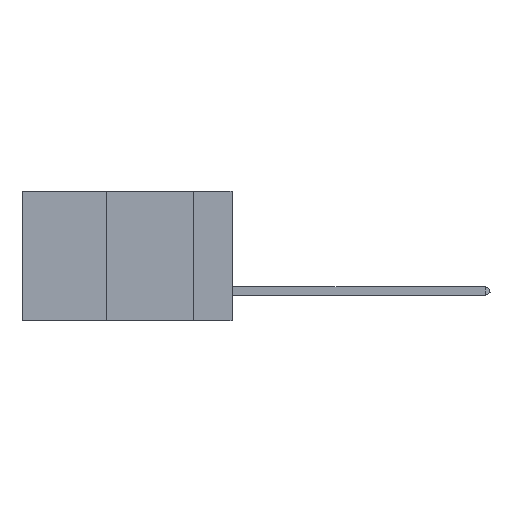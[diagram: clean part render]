
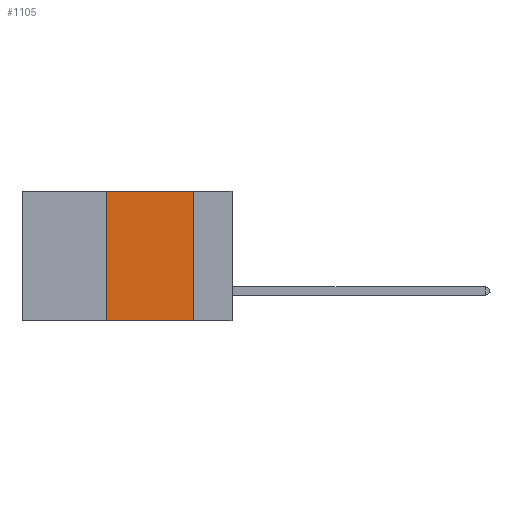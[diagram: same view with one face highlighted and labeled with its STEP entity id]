
A CAD part, left-side view. The second image highlights one B-rep face of the part: STEP entity #1105.
In plain terms, the highlighted planar face has unit normal (-1, 0, 0).
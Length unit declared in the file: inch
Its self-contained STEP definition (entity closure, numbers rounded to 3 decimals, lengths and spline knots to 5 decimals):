
#771 = CARTESIAN_POINT ( 'NONE',  ( 0., 0.6, -0.37 ) ) ;
#1045 = DIRECTION ( 'NONE',  ( 0., -1., 0. ) ) ;
#1105 = ADVANCED_FACE ( 'NONE', ( #7462 ), #9928, .F. ) ;
#1287 = CARTESIAN_POINT ( 'NONE',  ( 0., 0.36, 0. ) ) ;
#2020 = VERTEX_POINT ( 'NONE', #13612 ) ;
#2032 = CARTESIAN_POINT ( 'NONE',  ( 0., 0.11, -0.37 ) ) ;
#2173 = CARTESIAN_POINT ( 'NONE',  ( 0., 0.6, 0. ) ) ;
#2353 = LINE ( 'NONE', #771, #10437 ) ;
#2858 = DIRECTION ( 'NONE',  ( 0., 0., -1. ) ) ;
#2877 = EDGE_LOOP ( 'NONE', ( #5873, #17197, #14818, #10305 ) ) ;
#3292 = EDGE_CURVE ( 'NONE', #16500, #18222, #6842, .T. ) ;
#4449 = EDGE_CURVE ( 'NONE', #2020, #13318, #2353, .T. ) ;
#5873 = ORIENTED_EDGE ( 'NONE', *, *, #10106, .F. ) ;
#6842 = LINE ( 'NONE', #2173, #13228 ) ;
#7257 = DIRECTION ( 'NONE',  ( 0., 0., 1. ) ) ;
#7462 = FACE_OUTER_BOUND ( 'NONE', #2877, .T. ) ;
#9643 = DIRECTION ( 'NONE',  ( 0., 0., -1. ) ) ;
#9647 = AXIS2_PLACEMENT_3D ( 'NONE', #15613, #13117, #2858 ) ;
#9825 = VECTOR ( 'NONE', #7257, 39.37008 ) ;
#9928 = PLANE ( 'NONE',  #9647 ) ;
#10106 = EDGE_CURVE ( 'NONE', #18222, #13318, #11115, .T. ) ;
#10305 = ORIENTED_EDGE ( 'NONE', *, *, #4449, .T. ) ;
#10437 = VECTOR ( 'NONE', #1045, 39.37008 ) ;
#11115 = LINE ( 'NONE', #14024, #12352 ) ;
#12352 = VECTOR ( 'NONE', #9643, 39.37008 ) ;
#12861 = DIRECTION ( 'NONE',  ( 0., -1., 0. ) ) ;
#13117 = DIRECTION ( 'NONE',  ( 1., 0., 0. ) ) ;
#13228 = VECTOR ( 'NONE', #12861, 39.37008 ) ;
#13318 = VERTEX_POINT ( 'NONE', #2032 ) ;
#13612 = CARTESIAN_POINT ( 'NONE',  ( 0., 0.36, -0.37 ) ) ;
#13953 = CARTESIAN_POINT ( 'NONE',  ( 0., 0.11, 0. ) ) ;
#14024 = CARTESIAN_POINT ( 'NONE',  ( 0., 0.11, 0. ) ) ;
#14493 = LINE ( 'NONE', #16988, #9825 ) ;
#14818 = ORIENTED_EDGE ( 'NONE', *, *, #15791, .F. ) ;
#15613 = CARTESIAN_POINT ( 'NONE',  ( 0., 0.6, 0. ) ) ;
#15791 = EDGE_CURVE ( 'NONE', #2020, #16500, #14493, .T. ) ;
#16500 = VERTEX_POINT ( 'NONE', #1287 ) ;
#16988 = CARTESIAN_POINT ( 'NONE',  ( 0., 0.36, 0. ) ) ;
#17197 = ORIENTED_EDGE ( 'NONE', *, *, #3292, .F. ) ;
#18222 = VERTEX_POINT ( 'NONE', #13953 ) ;
